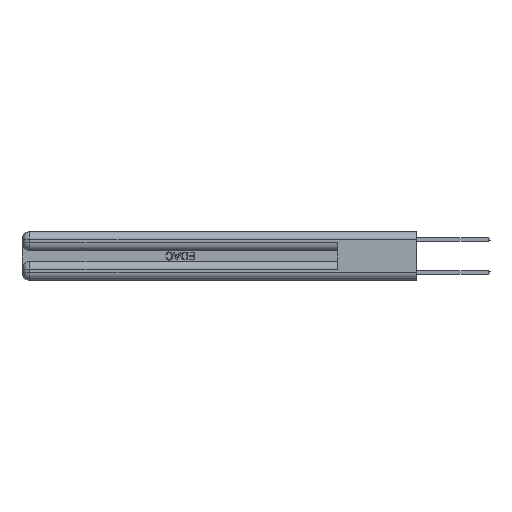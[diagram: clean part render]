
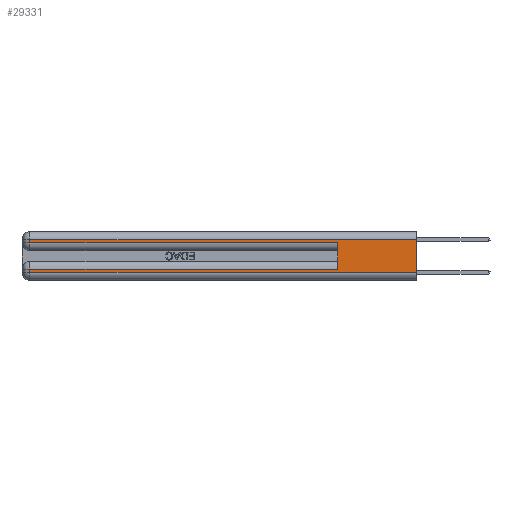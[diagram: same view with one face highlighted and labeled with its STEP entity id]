
A CAD part, left-side view. The second image highlights one B-rep face of the part: STEP entity #29331.
In plain terms, the highlighted planar face has unit normal (-1, 0, 0).
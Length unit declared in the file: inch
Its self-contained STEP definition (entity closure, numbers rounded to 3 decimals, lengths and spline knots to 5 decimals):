
#133 = CARTESIAN_POINT ( 'NONE',  ( 0., 0., 0.085 ) ) ;
#309 = LINE ( 'NONE', #133, #26138 ) ;
#961 = CARTESIAN_POINT ( 'NONE',  ( 0., 2.94, 0.31 ) ) ;
#995 = ORIENTED_EDGE ( 'NONE', *, *, #15609, .T. ) ;
#1539 = AXIS2_PLACEMENT_3D ( 'NONE', #4656, #28156, #14837 ) ;
#2242 = VECTOR ( 'NONE', #17559, 39.37008 ) ;
#2783 = ORIENTED_EDGE ( 'NONE', *, *, #17780, .F. ) ;
#4367 = VECTOR ( 'NONE', #29260, 39.37008 ) ;
#4656 = CARTESIAN_POINT ( 'NONE',  ( 0., 0., 0.37 ) ) ;
#4741 = CARTESIAN_POINT ( 'NONE',  ( 0., 0., 0.06 ) ) ;
#5153 = CARTESIAN_POINT ( 'NONE',  ( 0., 2.94, 0.37 ) ) ;
#5256 = VERTEX_POINT ( 'NONE', #4741 ) ;
#5882 = ORIENTED_EDGE ( 'NONE', *, *, #17582, .T. ) ;
#6871 = LINE ( 'NONE', #21630, #2242 ) ;
#7428 = VERTEX_POINT ( 'NONE', #34593 ) ;
#7606 = LINE ( 'NONE', #34387, #8833 ) ;
#8292 = CARTESIAN_POINT ( 'NONE',  ( 0., 0., 0.06 ) ) ;
#8814 = DIRECTION ( 'NONE',  ( 0., -1., 0. ) ) ;
#8833 = VECTOR ( 'NONE', #15842, 39.37008 ) ;
#10056 = EDGE_LOOP ( 'NONE', ( #18599, #5882, #995, #15804, #2783, #18589, #14411, #26067 ) ) ;
#10451 = DIRECTION ( 'NONE',  ( 0., 1., 0. ) ) ;
#10874 = CARTESIAN_POINT ( 'NONE',  ( 0., 2.94, 0.37 ) ) ;
#11235 = EDGE_CURVE ( 'NONE', #7428, #20201, #309, .T. ) ;
#12549 = VERTEX_POINT ( 'NONE', #19089 ) ;
#14063 = LINE ( 'NONE', #8292, #19290 ) ;
#14411 = ORIENTED_EDGE ( 'NONE', *, *, #25731, .T. ) ;
#14837 = DIRECTION ( 'NONE',  ( 0., 0., -1. ) ) ;
#15111 = EDGE_CURVE ( 'NONE', #16851, #19656, #7606, .T. ) ;
#15609 = EDGE_CURVE ( 'NONE', #32798, #16851, #26966, .T. ) ;
#15804 = ORIENTED_EDGE ( 'NONE', *, *, #15111, .T. ) ;
#15842 = DIRECTION ( 'NONE',  ( 0., -1., 0. ) ) ;
#15878 = DIRECTION ( 'NONE',  ( 0., 0., -1. ) ) ;
#16230 = CARTESIAN_POINT ( 'NONE',  ( 0., 0., 0.31 ) ) ;
#16851 = VERTEX_POINT ( 'NONE', #16999 ) ;
#16899 = CARTESIAN_POINT ( 'NONE',  ( 0., 0.6, 0.285 ) ) ;
#16999 = CARTESIAN_POINT ( 'NONE',  ( 0., 2.94, 0.285 ) ) ;
#17559 = DIRECTION ( 'NONE',  ( 0., 0., 1. ) ) ;
#17582 = EDGE_CURVE ( 'NONE', #25699, #32798, #29525, .T. ) ;
#17780 = EDGE_CURVE ( 'NONE', #7428, #19656, #6871, .T. ) ;
#18133 = EDGE_CURVE ( 'NONE', #25699, #5256, #22068, .T. ) ;
#18589 = ORIENTED_EDGE ( 'NONE', *, *, #11235, .T. ) ;
#18599 = ORIENTED_EDGE ( 'NONE', *, *, #18133, .F. ) ;
#19089 = CARTESIAN_POINT ( 'NONE',  ( 0., 2.94, 0.06 ) ) ;
#19290 = VECTOR ( 'NONE', #8814, 39.37008 ) ;
#19656 = VERTEX_POINT ( 'NONE', #16899 ) ;
#20201 = VERTEX_POINT ( 'NONE', #24208 ) ;
#20271 = FACE_OUTER_BOUND ( 'NONE', #10056, .T. ) ;
#21630 = CARTESIAN_POINT ( 'NONE',  ( 0., 0.6, 0.145 ) ) ;
#21698 = DIRECTION ( 'NONE',  ( 0., 1., 0. ) ) ;
#21771 = VECTOR ( 'NONE', #10451, 39.37008 ) ;
#22068 = LINE ( 'NONE', #27501, #33555 ) ;
#24208 = CARTESIAN_POINT ( 'NONE',  ( 0., 2.94, 0.085 ) ) ;
#25407 = DIRECTION ( 'NONE',  ( 0., 0., -1. ) ) ;
#25699 = VERTEX_POINT ( 'NONE', #31630 ) ;
#25731 = EDGE_CURVE ( 'NONE', #20201, #12549, #29173, .T. ) ;
#25877 = PLANE ( 'NONE',  #1539 ) ;
#26067 = ORIENTED_EDGE ( 'NONE', *, *, #27639, .T. ) ;
#26138 = VECTOR ( 'NONE', #21698, 39.37008 ) ;
#26966 = LINE ( 'NONE', #10874, #4367 ) ;
#27501 = CARTESIAN_POINT ( 'NONE',  ( 0., 0., 0.37 ) ) ;
#27639 = EDGE_CURVE ( 'NONE', #12549, #5256, #14063, .T. ) ;
#28156 = DIRECTION ( 'NONE',  ( 1., 0., 0. ) ) ;
#29173 = LINE ( 'NONE', #5153, #33222 ) ;
#29260 = DIRECTION ( 'NONE',  ( 0., 0., -1. ) ) ;
#29331 = ADVANCED_FACE ( 'NONE', ( #20271 ), #25877, .F. ) ;
#29525 = LINE ( 'NONE', #16230, #21771 ) ;
#31630 = CARTESIAN_POINT ( 'NONE',  ( 0., 0., 0.31 ) ) ;
#32798 = VERTEX_POINT ( 'NONE', #961 ) ;
#33222 = VECTOR ( 'NONE', #15878, 39.37008 ) ;
#33555 = VECTOR ( 'NONE', #25407, 39.37008 ) ;
#34387 = CARTESIAN_POINT ( 'NONE',  ( 0., 0., 0.285 ) ) ;
#34593 = CARTESIAN_POINT ( 'NONE',  ( 0., 0.6, 0.085 ) ) ;
